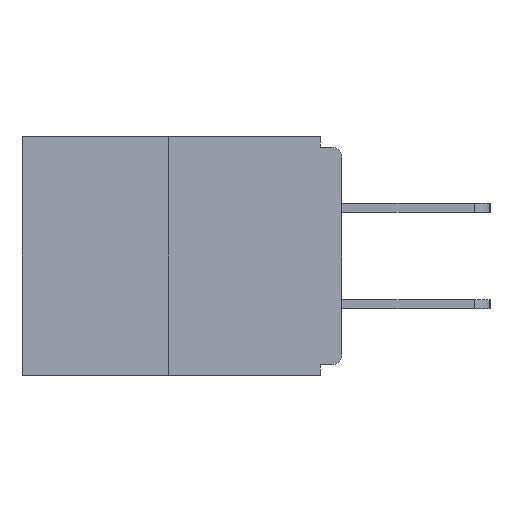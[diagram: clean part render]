
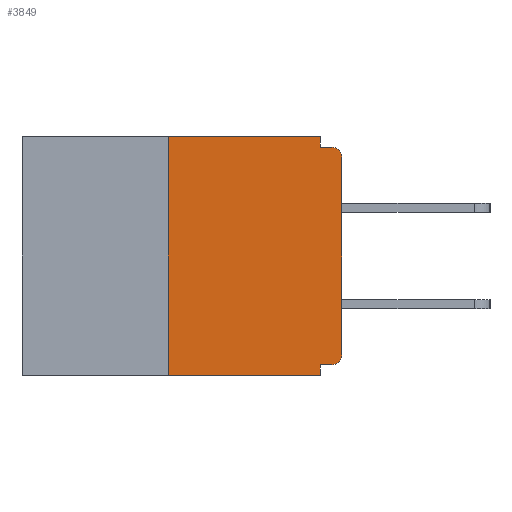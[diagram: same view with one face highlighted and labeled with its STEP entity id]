
A CAD part, left-side view. The second image highlights one B-rep face of the part: STEP entity #3849.
In plain terms, the highlighted planar face has unit normal (-1, 0, 0).
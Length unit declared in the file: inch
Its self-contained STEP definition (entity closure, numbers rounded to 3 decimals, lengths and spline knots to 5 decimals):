
#4 = EDGE_CURVE ( 'NONE', #557, #1018, #10783, .T. ) ;
#142 = DIRECTION ( 'NONE',  ( 0., 0., -1. ) ) ;
#236 = ORIENTED_EDGE ( 'NONE', *, *, #22929, .T. ) ;
#557 = VERTEX_POINT ( 'NONE', #18503 ) ;
#642 = EDGE_LOOP ( 'NONE', ( #6291, #5275, #8830, #8347, #14968, #13192, #236, #13669, #15230, #21221 ) ) ;
#906 = VERTEX_POINT ( 'NONE', #5259 ) ;
#1018 = VERTEX_POINT ( 'NONE', #26019 ) ;
#1349 = DIRECTION ( 'NONE',  ( 0., 0., -1. ) ) ;
#1367 = LINE ( 'NONE', #9602, #15541 ) ;
#1413 = VECTOR ( 'NONE', #25637, 39.37008 ) ;
#1691 = DIRECTION ( 'NONE',  ( 0., 0., -1. ) ) ;
#2053 = LINE ( 'NONE', #5512, #24246 ) ;
#2347 = VECTOR ( 'NONE', #16503, 39.37008 ) ;
#3013 = VECTOR ( 'NONE', #15539, 39.37008 ) ;
#3131 = EDGE_CURVE ( 'NONE', #9220, #16735, #14369, .T. ) ;
#3517 = DIRECTION ( 'NONE',  ( 0., 0., 1. ) ) ;
#3849 = ADVANCED_FACE ( 'NONE', ( #23291 ), #4617, .F. ) ;
#4617 = PLANE ( 'NONE',  #4710 ) ;
#4710 = AXIS2_PLACEMENT_3D ( 'NONE', #19099, #25287, #13032 ) ;
#4944 = EDGE_CURVE ( 'NONE', #20668, #557, #21983, .T. ) ;
#5166 = EDGE_CURVE ( 'NONE', #15045, #16735, #7491, .T. ) ;
#5251 = VERTEX_POINT ( 'NONE', #16244 ) ;
#5259 = CARTESIAN_POINT ( 'NONE',  ( 0., 0.015, -0.015 ) ) ;
#5275 = ORIENTED_EDGE ( 'NONE', *, *, #9322, .F. ) ;
#5512 = CARTESIAN_POINT ( 'NONE',  ( 0., 0., -0.328 ) ) ;
#6291 = ORIENTED_EDGE ( 'NONE', *, *, #4944, .F. ) ;
#6699 = EDGE_CURVE ( 'NONE', #16709, #906, #9012, .T. ) ;
#7491 = LINE ( 'NONE', #22778, #2347 ) ;
#8347 = ORIENTED_EDGE ( 'NONE', *, *, #3131, .F. ) ;
#8795 = EDGE_CURVE ( 'NONE', #1018, #906, #9797, .T. ) ;
#8830 = ORIENTED_EDGE ( 'NONE', *, *, #5166, .T. ) ;
#9012 = CIRCLE ( 'NONE', #18533, 0.015 ) ;
#9220 = VERTEX_POINT ( 'NONE', #10982 ) ;
#9322 = EDGE_CURVE ( 'NONE', #15045, #20668, #24547, .T. ) ;
#9602 = CARTESIAN_POINT ( 'NONE',  ( 0., 0., 0. ) ) ;
#9797 = LINE ( 'NONE', #22413, #24866 ) ;
#9957 = DIRECTION ( 'NONE',  ( 0., -1., 0. ) ) ;
#10783 = LINE ( 'NONE', #15743, #13354 ) ;
#10982 = CARTESIAN_POINT ( 'NONE',  ( 0., 0.031, -0.328 ) ) ;
#11042 = CARTESIAN_POINT ( 'NONE',  ( 0., 0.015, -0.313 ) ) ;
#11699 = DIRECTION ( 'NONE',  ( 0., 1., 0. ) ) ;
#12368 = CARTESIAN_POINT ( 'NONE',  ( 0., 0.031, -0.343 ) ) ;
#13032 = DIRECTION ( 'NONE',  ( 0., 0., -1. ) ) ;
#13192 = ORIENTED_EDGE ( 'NONE', *, *, #25083, .T. ) ;
#13354 = VECTOR ( 'NONE', #1349, 39.37008 ) ;
#13433 = CARTESIAN_POINT ( 'NONE',  ( 0., 0.25, 0. ) ) ;
#13669 = ORIENTED_EDGE ( 'NONE', *, *, #6699, .T. ) ;
#14369 = LINE ( 'NONE', #12368, #25238 ) ;
#14968 = ORIENTED_EDGE ( 'NONE', *, *, #21907, .F. ) ;
#15045 = VERTEX_POINT ( 'NONE', #16554 ) ;
#15230 = ORIENTED_EDGE ( 'NONE', *, *, #8795, .F. ) ;
#15240 = DIRECTION ( 'NONE',  ( 0., 0., -1. ) ) ;
#15539 = DIRECTION ( 'NONE',  ( 0., 0., 1. ) ) ;
#15541 = VECTOR ( 'NONE', #3517, 39.37008 ) ;
#15625 = CARTESIAN_POINT ( 'NONE',  ( 0., 0.25, 0. ) ) ;
#15743 = CARTESIAN_POINT ( 'NONE',  ( 0., 0.031, 0. ) ) ;
#15787 = CARTESIAN_POINT ( 'NONE',  ( 0., 0., -0.03 ) ) ;
#16244 = CARTESIAN_POINT ( 'NONE',  ( 0., 0., -0.313 ) ) ;
#16503 = DIRECTION ( 'NONE',  ( 0., -1., 0. ) ) ;
#16554 = CARTESIAN_POINT ( 'NONE',  ( 0., 0.25, -0.343 ) ) ;
#16709 = VERTEX_POINT ( 'NONE', #15787 ) ;
#16735 = VERTEX_POINT ( 'NONE', #17904 ) ;
#17107 = DIRECTION ( 'NONE',  ( -1., 0., 0. ) ) ;
#17691 = VERTEX_POINT ( 'NONE', #23134 ) ;
#17904 = CARTESIAN_POINT ( 'NONE',  ( 0., 0.031, -0.343 ) ) ;
#18000 = AXIS2_PLACEMENT_3D ( 'NONE', #11042, #17107, #15240 ) ;
#18131 = DIRECTION ( 'NONE',  ( -1., 0., 0. ) ) ;
#18503 = CARTESIAN_POINT ( 'NONE',  ( 0., 0.031, 0. ) ) ;
#18533 = AXIS2_PLACEMENT_3D ( 'NONE', #19863, #18131, #1691 ) ;
#19099 = CARTESIAN_POINT ( 'NONE',  ( 0., 0.46, 0. ) ) ;
#19863 = CARTESIAN_POINT ( 'NONE',  ( 0., 0.015, -0.03 ) ) ;
#20668 = VERTEX_POINT ( 'NONE', #13433 ) ;
#21221 = ORIENTED_EDGE ( 'NONE', *, *, #4, .F. ) ;
#21907 = EDGE_CURVE ( 'NONE', #17691, #9220, #2053, .T. ) ;
#21983 = LINE ( 'NONE', #23670, #1413 ) ;
#22413 = CARTESIAN_POINT ( 'NONE',  ( 0., 0., -0.015 ) ) ;
#22778 = CARTESIAN_POINT ( 'NONE',  ( 0., 0.46, -0.343 ) ) ;
#22929 = EDGE_CURVE ( 'NONE', #5251, #16709, #1367, .T. ) ;
#23134 = CARTESIAN_POINT ( 'NONE',  ( 0., 0.015, -0.328 ) ) ;
#23291 = FACE_OUTER_BOUND ( 'NONE', #642, .T. ) ;
#23670 = CARTESIAN_POINT ( 'NONE',  ( 0., 0.46, 0. ) ) ;
#24094 = CIRCLE ( 'NONE', #18000, 0.015 ) ;
#24246 = VECTOR ( 'NONE', #11699, 39.37008 ) ;
#24547 = LINE ( 'NONE', #15625, #3013 ) ;
#24866 = VECTOR ( 'NONE', #9957, 39.37008 ) ;
#25083 = EDGE_CURVE ( 'NONE', #17691, #5251, #24094, .T. ) ;
#25238 = VECTOR ( 'NONE', #142, 39.37008 ) ;
#25287 = DIRECTION ( 'NONE',  ( 1., 0., 0. ) ) ;
#25637 = DIRECTION ( 'NONE',  ( 0., -1., 0. ) ) ;
#26019 = CARTESIAN_POINT ( 'NONE',  ( 0., 0.031, -0.015 ) ) ;
